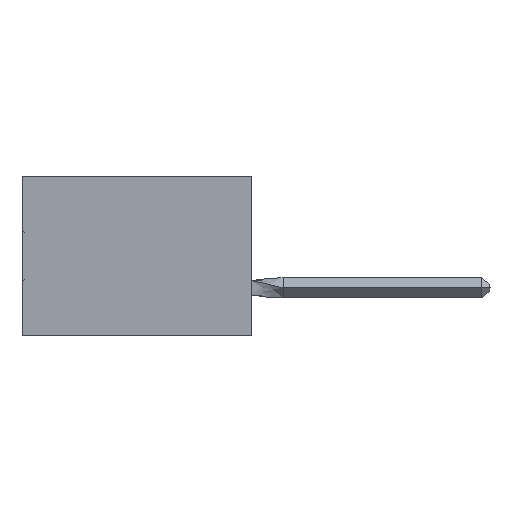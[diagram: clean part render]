
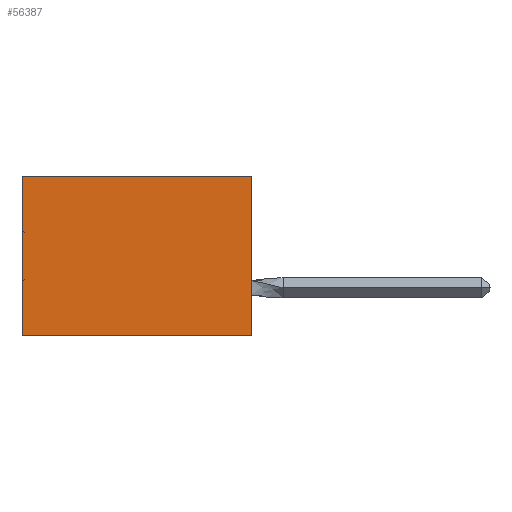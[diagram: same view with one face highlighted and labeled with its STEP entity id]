
A CAD part, left-side view. The second image highlights one B-rep face of the part: STEP entity #56387.
In plain terms, the highlighted planar face has unit normal (-1, 0, 0).
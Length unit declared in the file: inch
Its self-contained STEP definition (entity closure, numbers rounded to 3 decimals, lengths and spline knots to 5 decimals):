
#3353 = CARTESIAN_POINT ( 'NONE',  ( 0.305, 0.72, -0.5 ) ) ;
#3954 = VERTEX_POINT ( 'NONE', #50895 ) ;
#4214 = ORIENTED_EDGE ( 'NONE', *, *, #25593, .F. ) ;
#8803 = LINE ( 'NONE', #9882, #20378 ) ;
#9882 = CARTESIAN_POINT ( 'NONE',  ( 0.305, 0., -0.5 ) ) ;
#10167 = CARTESIAN_POINT ( 'NONE',  ( 0.305, 0., 0. ) ) ;
#10570 = EDGE_CURVE ( 'NONE', #25948, #29771, #8803, .T. ) ;
#11912 = EDGE_CURVE ( 'NONE', #14047, #3954, #45580, .T. ) ;
#12001 = EDGE_CURVE ( 'NONE', #3954, #29771, #40813, .T. ) ;
#12686 = VECTOR ( 'NONE', #16327, 39.37008 ) ;
#13557 = ORIENTED_EDGE ( 'NONE', *, *, #10570, .F. ) ;
#14047 = VERTEX_POINT ( 'NONE', #10167 ) ;
#14814 = DIRECTION ( 'NONE',  ( 1., 0., 0. ) ) ;
#15307 = LINE ( 'NONE', #31915, #19442 ) ;
#16327 = DIRECTION ( 'NONE',  ( 0., 0., -1. ) ) ;
#19442 = VECTOR ( 'NONE', #36322, 39.37008 ) ;
#20378 = VECTOR ( 'NONE', #52895, 39.37008 ) ;
#23288 = CARTESIAN_POINT ( 'NONE',  ( 0.305, 0., -0.5 ) ) ;
#25593 = EDGE_CURVE ( 'NONE', #14047, #25948, #15307, .T. ) ;
#25948 = VERTEX_POINT ( 'NONE', #27730 ) ;
#26550 = FACE_OUTER_BOUND ( 'NONE', #32714, .T. ) ;
#27730 = CARTESIAN_POINT ( 'NONE',  ( 0.305, 0., -0.5 ) ) ;
#29571 = CARTESIAN_POINT ( 'NONE',  ( 0.305, 0., 0. ) ) ;
#29771 = VERTEX_POINT ( 'NONE', #55376 ) ;
#31915 = CARTESIAN_POINT ( 'NONE',  ( 0.305, 0., -0.5 ) ) ;
#31929 = VECTOR ( 'NONE', #51676, 39.37008 ) ;
#32506 = PLANE ( 'NONE',  #45414 ) ;
#32714 = EDGE_LOOP ( 'NONE', ( #42450, #13557, #4214, #33010 ) ) ;
#33010 = ORIENTED_EDGE ( 'NONE', *, *, #11912, .T. ) ;
#36322 = DIRECTION ( 'NONE',  ( 0., 0., -1. ) ) ;
#40813 = LINE ( 'NONE', #3353, #12686 ) ;
#42450 = ORIENTED_EDGE ( 'NONE', *, *, #12001, .T. ) ;
#45414 = AXIS2_PLACEMENT_3D ( 'NONE', #23288, #14814, #45444 ) ;
#45444 = DIRECTION ( 'NONE',  ( 0., 0., -1. ) ) ;
#45580 = LINE ( 'NONE', #29571, #31929 ) ;
#50895 = CARTESIAN_POINT ( 'NONE',  ( 0.305, 0.72, 0. ) ) ;
#51676 = DIRECTION ( 'NONE',  ( 0., 1., 0. ) ) ;
#52895 = DIRECTION ( 'NONE',  ( 0., 1., 0. ) ) ;
#55376 = CARTESIAN_POINT ( 'NONE',  ( 0.305, 0.72, -0.5 ) ) ;
#56387 = ADVANCED_FACE ( 'NONE', ( #26550 ), #32506, .F. ) ;
